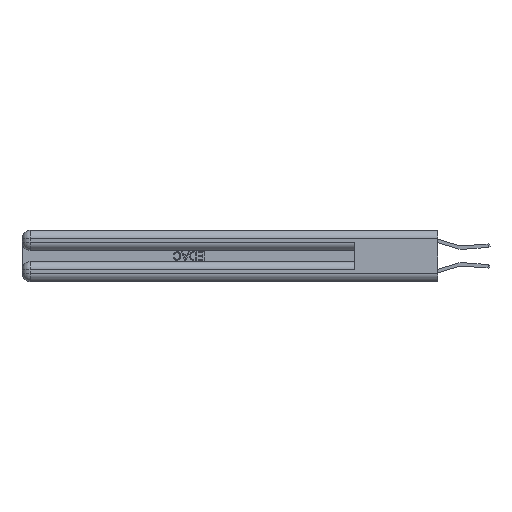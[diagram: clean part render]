
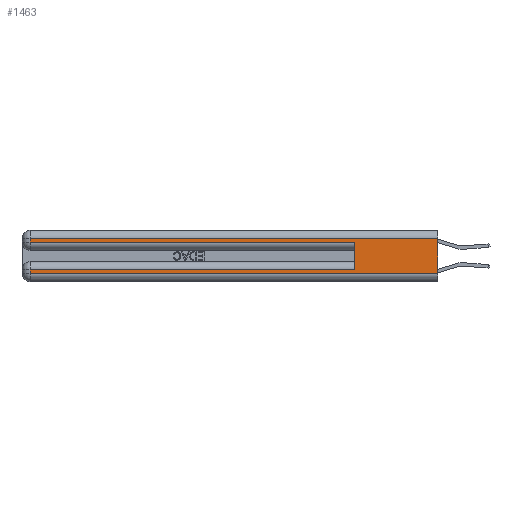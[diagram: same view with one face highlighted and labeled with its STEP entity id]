
A CAD part, left-side view. The second image highlights one B-rep face of the part: STEP entity #1463.
In plain terms, the highlighted planar face has unit normal (-1, 0, 0).
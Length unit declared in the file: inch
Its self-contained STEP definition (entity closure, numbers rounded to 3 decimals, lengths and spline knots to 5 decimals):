
#328 = EDGE_CURVE ( 'NONE', #12387, #26974, #18746, .T. ) ;
#596 = ORIENTED_EDGE ( 'NONE', *, *, #22534, .T. ) ;
#1004 = DIRECTION ( 'NONE',  ( 0., 0., -1. ) ) ;
#1055 = PLANE ( 'NONE',  #2959 ) ;
#1077 = EDGE_CURVE ( 'NONE', #26974, #25609, #25503, .T. ) ;
#1390 = CARTESIAN_POINT ( 'NONE',  ( 0., 0., 0.37 ) ) ;
#1463 = ADVANCED_FACE ( 'NONE', ( #16396 ), #1055, .F. ) ;
#1964 = VERTEX_POINT ( 'NONE', #9568 ) ;
#2063 = DIRECTION ( 'NONE',  ( 0., 0., -1. ) ) ;
#2080 = CARTESIAN_POINT ( 'NONE',  ( 0., 0., 0.06 ) ) ;
#2206 = DIRECTION ( 'NONE',  ( 0., 1., 0. ) ) ;
#2265 = ORIENTED_EDGE ( 'NONE', *, *, #5042, .F. ) ;
#2577 = VECTOR ( 'NONE', #22162, 39.37008 ) ;
#2707 = VERTEX_POINT ( 'NONE', #11974 ) ;
#2823 = VECTOR ( 'NONE', #3552, 39.37008 ) ;
#2959 = AXIS2_PLACEMENT_3D ( 'NONE', #5447, #16154, #26903 ) ;
#3552 = DIRECTION ( 'NONE',  ( 0., -1., 0. ) ) ;
#4282 = CARTESIAN_POINT ( 'NONE',  ( 0., 2.94, 0.37 ) ) ;
#5042 = EDGE_CURVE ( 'NONE', #12387, #9436, #8752, .T. ) ;
#5447 = CARTESIAN_POINT ( 'NONE',  ( 0., 0., 0.37 ) ) ;
#7534 = EDGE_CURVE ( 'NONE', #1964, #9436, #10709, .T. ) ;
#7715 = VECTOR ( 'NONE', #1004, 39.37008 ) ;
#8375 = LINE ( 'NONE', #26952, #2577 ) ;
#8567 = CARTESIAN_POINT ( 'NONE',  ( 0., 0.6, 0.285 ) ) ;
#8655 = CARTESIAN_POINT ( 'NONE',  ( 0., 2.94, 0.285 ) ) ;
#8752 = LINE ( 'NONE', #1390, #7715 ) ;
#9436 = VERTEX_POINT ( 'NONE', #25369 ) ;
#9568 = CARTESIAN_POINT ( 'NONE',  ( 0., 2.94, 0.06 ) ) ;
#9865 = ORIENTED_EDGE ( 'NONE', *, *, #7534, .T. ) ;
#9927 = LINE ( 'NONE', #15469, #22061 ) ;
#10100 = DIRECTION ( 'NONE',  ( 0., 0., -1. ) ) ;
#10709 = LINE ( 'NONE', #2080, #17793 ) ;
#11957 = VERTEX_POINT ( 'NONE', #20179 ) ;
#11974 = CARTESIAN_POINT ( 'NONE',  ( 0., 2.94, 0.085 ) ) ;
#12387 = VERTEX_POINT ( 'NONE', #22070 ) ;
#13720 = EDGE_CURVE ( 'NONE', #11957, #2707, #9927, .T. ) ;
#13925 = ORIENTED_EDGE ( 'NONE', *, *, #328, .T. ) ;
#14244 = ORIENTED_EDGE ( 'NONE', *, *, #15292, .T. ) ;
#14362 = LINE ( 'NONE', #23013, #2823 ) ;
#14385 = VECTOR ( 'NONE', #10100, 39.37008 ) ;
#14701 = VECTOR ( 'NONE', #2206, 39.37008 ) ;
#15292 = EDGE_CURVE ( 'NONE', #2707, #1964, #16904, .T. ) ;
#15428 = CARTESIAN_POINT ( 'NONE',  ( 0., 2.94, 0.31 ) ) ;
#15469 = CARTESIAN_POINT ( 'NONE',  ( 0., 0., 0.085 ) ) ;
#16154 = DIRECTION ( 'NONE',  ( 1., 0., 0. ) ) ;
#16250 = VECTOR ( 'NONE', #2063, 39.37008 ) ;
#16396 = FACE_OUTER_BOUND ( 'NONE', #25934, .T. ) ;
#16904 = LINE ( 'NONE', #4282, #16250 ) ;
#17793 = VECTOR ( 'NONE', #21747, 39.37008 ) ;
#17808 = ORIENTED_EDGE ( 'NONE', *, *, #1077, .T. ) ;
#18746 = LINE ( 'NONE', #19706, #14701 ) ;
#19706 = CARTESIAN_POINT ( 'NONE',  ( 0., 0., 0.31 ) ) ;
#20179 = CARTESIAN_POINT ( 'NONE',  ( 0., 0.6, 0.085 ) ) ;
#20943 = EDGE_CURVE ( 'NONE', #11957, #21111, #8375, .T. ) ;
#21111 = VERTEX_POINT ( 'NONE', #8567 ) ;
#21587 = ORIENTED_EDGE ( 'NONE', *, *, #13720, .T. ) ;
#21747 = DIRECTION ( 'NONE',  ( 0., -1., 0. ) ) ;
#22061 = VECTOR ( 'NONE', #26046, 39.37008 ) ;
#22070 = CARTESIAN_POINT ( 'NONE',  ( 0., 0., 0.31 ) ) ;
#22162 = DIRECTION ( 'NONE',  ( 0., 0., 1. ) ) ;
#22534 = EDGE_CURVE ( 'NONE', #25609, #21111, #14362, .T. ) ;
#23013 = CARTESIAN_POINT ( 'NONE',  ( 0., 0., 0.285 ) ) ;
#23185 = ORIENTED_EDGE ( 'NONE', *, *, #20943, .F. ) ;
#25369 = CARTESIAN_POINT ( 'NONE',  ( 0., 0., 0.06 ) ) ;
#25503 = LINE ( 'NONE', #27296, #14385 ) ;
#25609 = VERTEX_POINT ( 'NONE', #8655 ) ;
#25934 = EDGE_LOOP ( 'NONE', ( #2265, #13925, #17808, #596, #23185, #21587, #14244, #9865 ) ) ;
#26046 = DIRECTION ( 'NONE',  ( 0., 1., 0. ) ) ;
#26903 = DIRECTION ( 'NONE',  ( 0., 0., -1. ) ) ;
#26952 = CARTESIAN_POINT ( 'NONE',  ( 0., 0.6, 0.145 ) ) ;
#26974 = VERTEX_POINT ( 'NONE', #15428 ) ;
#27296 = CARTESIAN_POINT ( 'NONE',  ( 0., 2.94, 0.37 ) ) ;
